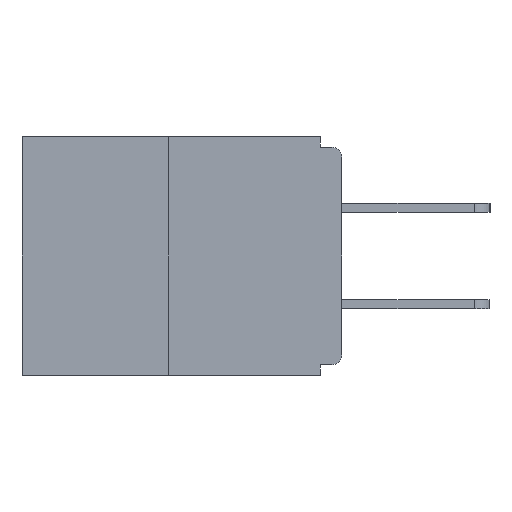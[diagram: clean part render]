
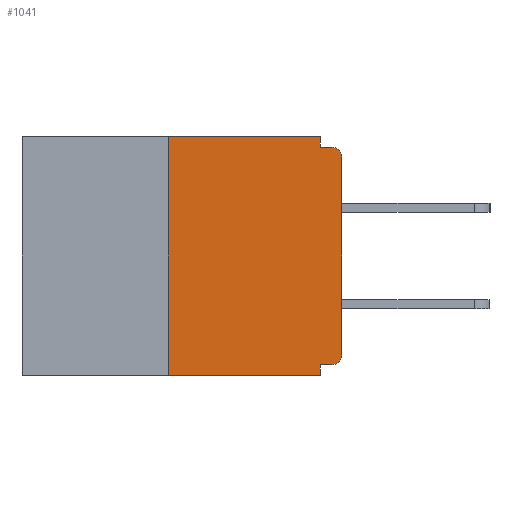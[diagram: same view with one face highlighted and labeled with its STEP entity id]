
A CAD part, left-side view. The second image highlights one B-rep face of the part: STEP entity #1041.
In plain terms, the highlighted planar face has unit normal (-1, 0, 0).
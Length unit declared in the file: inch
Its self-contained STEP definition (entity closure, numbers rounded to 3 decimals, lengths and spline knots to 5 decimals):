
#64 = CARTESIAN_POINT ( 'NONE',  ( 0., 0., 0. ) ) ;
#202 = LINE ( 'NONE', #5916, #10474 ) ;
#384 = CARTESIAN_POINT ( 'NONE',  ( 0., 0.031, -0.328 ) ) ;
#464 = CIRCLE ( 'NONE', #8037, 0.015 ) ;
#486 = DIRECTION ( 'NONE',  ( -1., 0., 0. ) ) ;
#650 = EDGE_CURVE ( 'NONE', #12208, #2219, #8982, .T. ) ;
#732 = ORIENTED_EDGE ( 'NONE', *, *, #4322, .T. ) ;
#805 = VECTOR ( 'NONE', #3749, 39.37008 ) ;
#1041 = ADVANCED_FACE ( 'NONE', ( #5436 ), #5211, .F. ) ;
#1452 = VERTEX_POINT ( 'NONE', #8708 ) ;
#1609 = DIRECTION ( 'NONE',  ( -1., 0., 0. ) ) ;
#1743 = DIRECTION ( 'NONE',  ( 0., 0., -1. ) ) ;
#1836 = EDGE_CURVE ( 'NONE', #12620, #9768, #8643, .T. ) ;
#2219 = VERTEX_POINT ( 'NONE', #11523 ) ;
#2364 = ORIENTED_EDGE ( 'NONE', *, *, #650, .T. ) ;
#2372 = CARTESIAN_POINT ( 'NONE',  ( 0., 0., -0.03 ) ) ;
#2640 = VERTEX_POINT ( 'NONE', #384 ) ;
#2738 = ORIENTED_EDGE ( 'NONE', *, *, #8688, .F. ) ;
#2836 = CARTESIAN_POINT ( 'NONE',  ( 0., 0.031, 0. ) ) ;
#2926 = DIRECTION ( 'NONE',  ( 0., 0., 1. ) ) ;
#2969 = EDGE_CURVE ( 'NONE', #5654, #2640, #8620, .T. ) ;
#3412 = DIRECTION ( 'NONE',  ( 0., -1., 0. ) ) ;
#3568 = CARTESIAN_POINT ( 'NONE',  ( 0., 0.015, -0.03 ) ) ;
#3583 = CARTESIAN_POINT ( 'NONE',  ( 0., 0.015, -0.313 ) ) ;
#3749 = DIRECTION ( 'NONE',  ( 0., 1., 0. ) ) ;
#3780 = EDGE_CURVE ( 'NONE', #5654, #12620, #464, .T. ) ;
#3828 = CIRCLE ( 'NONE', #7371, 0.015 ) ;
#4087 = VECTOR ( 'NONE', #3412, 39.37008 ) ;
#4280 = CARTESIAN_POINT ( 'NONE',  ( 0., 0., -0.015 ) ) ;
#4286 = DIRECTION ( 'NONE',  ( 0., -1., 0. ) ) ;
#4322 = EDGE_CURVE ( 'NONE', #9768, #7160, #3828, .T. ) ;
#4406 = CARTESIAN_POINT ( 'NONE',  ( 0., 0.46, -0.343 ) ) ;
#4600 = ORIENTED_EDGE ( 'NONE', *, *, #3780, .T. ) ;
#4617 = EDGE_CURVE ( 'NONE', #12511, #1452, #11787, .T. ) ;
#4810 = CARTESIAN_POINT ( 'NONE',  ( 0., 0., -0.313 ) ) ;
#5082 = CARTESIAN_POINT ( 'NONE',  ( 0., 0.25, -0.343 ) ) ;
#5211 = PLANE ( 'NONE',  #7659 ) ;
#5436 = FACE_OUTER_BOUND ( 'NONE', #5623, .T. ) ;
#5623 = EDGE_LOOP ( 'NONE', ( #10573, #2738, #2364, #8935, #9740, #4600, #10942, #732, #7971, #8264 ) ) ;
#5654 = VERTEX_POINT ( 'NONE', #11284 ) ;
#5916 = CARTESIAN_POINT ( 'NONE',  ( 0., 0.25, 0. ) ) ;
#6117 = CARTESIAN_POINT ( 'NONE',  ( 0., 0.031, -0.343 ) ) ;
#6192 = DIRECTION ( 'NONE',  ( 0., 0., -1. ) ) ;
#6210 = CARTESIAN_POINT ( 'NONE',  ( 0., 0.46, 0. ) ) ;
#6880 = DIRECTION ( 'NONE',  ( 0., 0., -1. ) ) ;
#7160 = VERTEX_POINT ( 'NONE', #11949 ) ;
#7238 = DIRECTION ( 'NONE',  ( 0., 0., -1. ) ) ;
#7289 = DIRECTION ( 'NONE',  ( 0., -1., 0. ) ) ;
#7371 = AXIS2_PLACEMENT_3D ( 'NONE', #3568, #486, #8333 ) ;
#7525 = VECTOR ( 'NONE', #4286, 39.37008 ) ;
#7536 = VECTOR ( 'NONE', #7289, 39.37008 ) ;
#7647 = CARTESIAN_POINT ( 'NONE',  ( 0., 0., -0.328 ) ) ;
#7659 = AXIS2_PLACEMENT_3D ( 'NONE', #8172, #10111, #6192 ) ;
#7748 = EDGE_CURVE ( 'NONE', #2640, #2219, #8050, .T. ) ;
#7753 = LINE ( 'NONE', #6210, #7525 ) ;
#7971 = ORIENTED_EDGE ( 'NONE', *, *, #10154, .F. ) ;
#8037 = AXIS2_PLACEMENT_3D ( 'NONE', #3583, #1609, #1743 ) ;
#8050 = LINE ( 'NONE', #6117, #11396 ) ;
#8172 = CARTESIAN_POINT ( 'NONE',  ( 0., 0.46, 0. ) ) ;
#8264 = ORIENTED_EDGE ( 'NONE', *, *, #4617, .F. ) ;
#8333 = DIRECTION ( 'NONE',  ( 0., 0., -1. ) ) ;
#8620 = LINE ( 'NONE', #7647, #805 ) ;
#8643 = LINE ( 'NONE', #64, #9541 ) ;
#8688 = EDGE_CURVE ( 'NONE', #12208, #9207, #202, .T. ) ;
#8708 = CARTESIAN_POINT ( 'NONE',  ( 0., 0.031, -0.015 ) ) ;
#8935 = ORIENTED_EDGE ( 'NONE', *, *, #7748, .F. ) ;
#8982 = LINE ( 'NONE', #4406, #4087 ) ;
#9207 = VERTEX_POINT ( 'NONE', #11415 ) ;
#9378 = CARTESIAN_POINT ( 'NONE',  ( 0., 0.031, 0. ) ) ;
#9541 = VECTOR ( 'NONE', #2926, 39.37008 ) ;
#9740 = ORIENTED_EDGE ( 'NONE', *, *, #2969, .F. ) ;
#9768 = VERTEX_POINT ( 'NONE', #2372 ) ;
#10111 = DIRECTION ( 'NONE',  ( 1., 0., 0. ) ) ;
#10154 = EDGE_CURVE ( 'NONE', #1452, #7160, #10437, .T. ) ;
#10241 = VECTOR ( 'NONE', #6880, 39.37008 ) ;
#10437 = LINE ( 'NONE', #4280, #7536 ) ;
#10474 = VECTOR ( 'NONE', #11872, 39.37008 ) ;
#10573 = ORIENTED_EDGE ( 'NONE', *, *, #11152, .F. ) ;
#10942 = ORIENTED_EDGE ( 'NONE', *, *, #1836, .T. ) ;
#11152 = EDGE_CURVE ( 'NONE', #9207, #12511, #7753, .T. ) ;
#11284 = CARTESIAN_POINT ( 'NONE',  ( 0., 0.015, -0.328 ) ) ;
#11396 = VECTOR ( 'NONE', #7238, 39.37008 ) ;
#11415 = CARTESIAN_POINT ( 'NONE',  ( 0., 0.25, 0. ) ) ;
#11523 = CARTESIAN_POINT ( 'NONE',  ( 0., 0.031, -0.343 ) ) ;
#11787 = LINE ( 'NONE', #2836, #10241 ) ;
#11872 = DIRECTION ( 'NONE',  ( 0., 0., 1. ) ) ;
#11949 = CARTESIAN_POINT ( 'NONE',  ( 0., 0.015, -0.015 ) ) ;
#12208 = VERTEX_POINT ( 'NONE', #5082 ) ;
#12511 = VERTEX_POINT ( 'NONE', #9378 ) ;
#12620 = VERTEX_POINT ( 'NONE', #4810 ) ;
